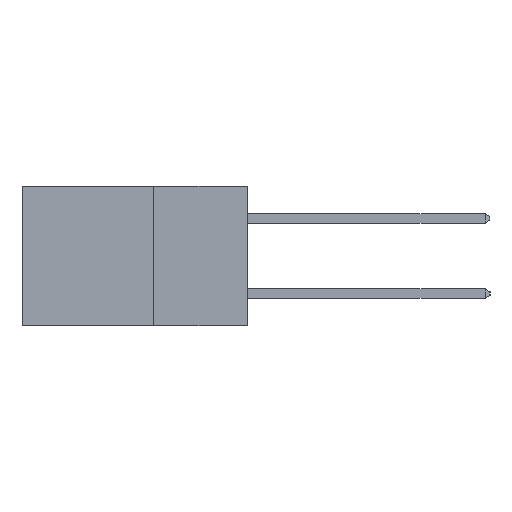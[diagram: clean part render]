
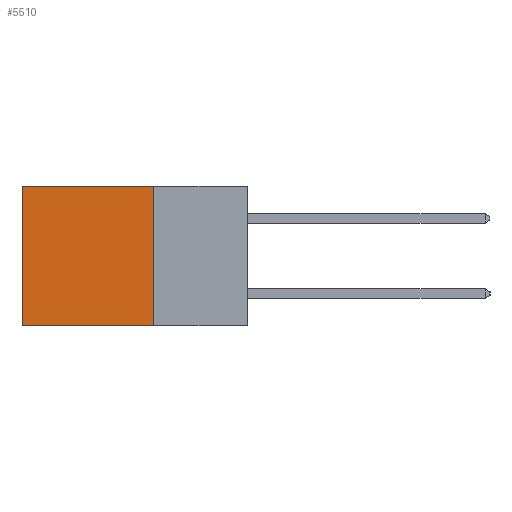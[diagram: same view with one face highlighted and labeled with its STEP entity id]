
A CAD part, left-side view. The second image highlights one B-rep face of the part: STEP entity #5510.
In plain terms, the highlighted planar face has unit normal (-1, 0, 0).
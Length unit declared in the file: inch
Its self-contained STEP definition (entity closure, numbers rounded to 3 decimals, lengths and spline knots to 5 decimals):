
#677 = LINE ( 'NONE', #9096, #8480 ) ;
#727 = VERTEX_POINT ( 'NONE', #11443 ) ;
#1214 = VERTEX_POINT ( 'NONE', #4600 ) ;
#1403 = FACE_OUTER_BOUND ( 'NONE', #7356, .T. ) ;
#1973 = LINE ( 'NONE', #8578, #6782 ) ;
#2109 = VERTEX_POINT ( 'NONE', #12267 ) ;
#2229 = VECTOR ( 'NONE', #6036, 39.37008 ) ;
#3509 = VERTEX_POINT ( 'NONE', #11031 ) ;
#4128 = ORIENTED_EDGE ( 'NONE', *, *, #4214, .T. ) ;
#4213 = VECTOR ( 'NONE', #12024, 39.37008 ) ;
#4214 = EDGE_CURVE ( 'NONE', #727, #1214, #10373, .T. ) ;
#4600 = CARTESIAN_POINT ( 'NONE',  ( 0.2615, 0.6, -0.37 ) ) ;
#4647 = DIRECTION ( 'NONE',  ( 1., 0., 0. ) ) ;
#4680 = DIRECTION ( 'NONE',  ( 0., 0., -1. ) ) ;
#4778 = CARTESIAN_POINT ( 'NONE',  ( 0.2615, 0.25, -0.37 ) ) ;
#4896 = PLANE ( 'NONE',  #7615 ) ;
#5510 = ADVANCED_FACE ( 'NONE', ( #1403 ), #4896, .F. ) ;
#5678 = EDGE_CURVE ( 'NONE', #3509, #727, #6991, .T. ) ;
#6036 = DIRECTION ( 'NONE',  ( 0., 0., -1. ) ) ;
#6349 = CARTESIAN_POINT ( 'NONE',  ( 0.2615, 0.6, -0.37 ) ) ;
#6782 = VECTOR ( 'NONE', #8361, 39.37008 ) ;
#6991 = LINE ( 'NONE', #12387, #4213 ) ;
#7356 = EDGE_LOOP ( 'NONE', ( #4128, #12078, #7598, #7726 ) ) ;
#7412 = EDGE_CURVE ( 'NONE', #2109, #1214, #1973, .T. ) ;
#7598 = ORIENTED_EDGE ( 'NONE', *, *, #8371, .F. ) ;
#7615 = AXIS2_PLACEMENT_3D ( 'NONE', #4778, #4647, #4680 ) ;
#7726 = ORIENTED_EDGE ( 'NONE', *, *, #5678, .T. ) ;
#8361 = DIRECTION ( 'NONE',  ( 0., 1., 0. ) ) ;
#8371 = EDGE_CURVE ( 'NONE', #3509, #2109, #677, .T. ) ;
#8480 = VECTOR ( 'NONE', #9576, 39.37008 ) ;
#8578 = CARTESIAN_POINT ( 'NONE',  ( 0.2615, 0.25, -0.37 ) ) ;
#9096 = CARTESIAN_POINT ( 'NONE',  ( 0.2615, 0.25, -0.37 ) ) ;
#9576 = DIRECTION ( 'NONE',  ( 0., 0., -1. ) ) ;
#10373 = LINE ( 'NONE', #6349, #2229 ) ;
#11031 = CARTESIAN_POINT ( 'NONE',  ( 0.2615, 0.25, 0. ) ) ;
#11443 = CARTESIAN_POINT ( 'NONE',  ( 0.2615, 0.6, 0. ) ) ;
#12024 = DIRECTION ( 'NONE',  ( 0., 1., 0. ) ) ;
#12078 = ORIENTED_EDGE ( 'NONE', *, *, #7412, .F. ) ;
#12267 = CARTESIAN_POINT ( 'NONE',  ( 0.2615, 0.25, -0.37 ) ) ;
#12387 = CARTESIAN_POINT ( 'NONE',  ( 0.2615, 0.25, 0. ) ) ;
